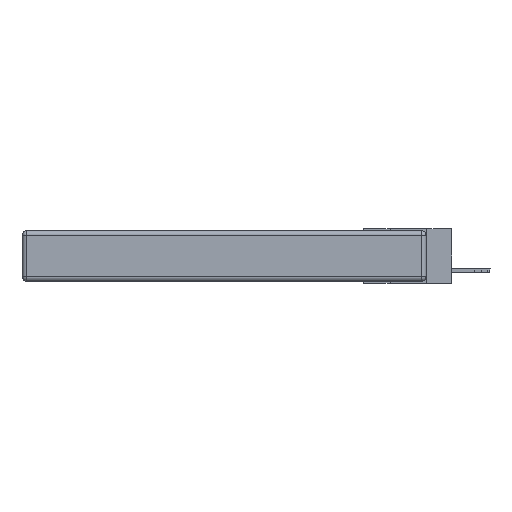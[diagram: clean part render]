
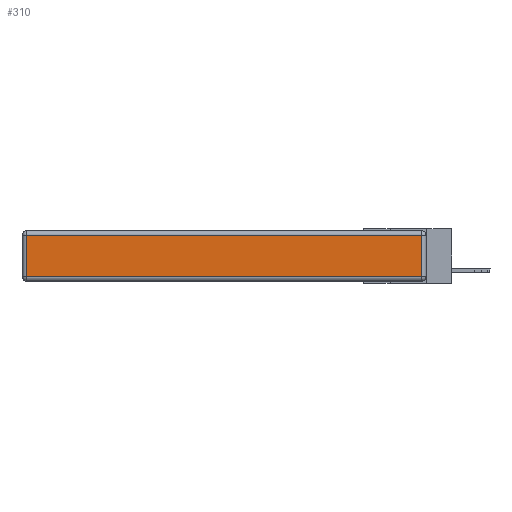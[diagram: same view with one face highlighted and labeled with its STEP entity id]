
A CAD part, left-side view. The second image highlights one B-rep face of the part: STEP entity #310.
In plain terms, the highlighted planar face has unit normal (-1, 0, 0).
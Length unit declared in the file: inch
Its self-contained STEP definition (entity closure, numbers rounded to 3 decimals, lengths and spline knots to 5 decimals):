
#116 = DIRECTION ( 'NONE',  ( 0., 1., 0. ) ) ;
#310 = ADVANCED_FACE ( 'NONE', ( #9126 ), #2979, .T. ) ;
#355 = DIRECTION ( 'NONE',  ( 0., 0., 1. ) ) ;
#733 = ORIENTED_EDGE ( 'NONE', *, *, #12509, .T. ) ;
#1388 = CARTESIAN_POINT ( 'NONE',  ( 0., 0.03, -0.03 ) ) ;
#1414 = ORIENTED_EDGE ( 'NONE', *, *, #11824, .T. ) ;
#1596 = VERTEX_POINT ( 'NONE', #8370 ) ;
#1909 = LINE ( 'NONE', #14400, #7045 ) ;
#2742 = CARTESIAN_POINT ( 'NONE',  ( 0., 0., -0.343 ) ) ;
#2979 = PLANE ( 'NONE',  #8669 ) ;
#3064 = EDGE_CURVE ( 'NONE', #5934, #12374, #6732, .T. ) ;
#3656 = CARTESIAN_POINT ( 'NONE',  ( 0., 2.72, -0.343 ) ) ;
#4066 = DIRECTION ( 'NONE',  ( -1., 0., 0. ) ) ;
#4663 = CARTESIAN_POINT ( 'NONE',  ( 0., 2.72, -0.03 ) ) ;
#4670 = ORIENTED_EDGE ( 'NONE', *, *, #5881, .T. ) ;
#5603 = LINE ( 'NONE', #5982, #16171 ) ;
#5881 = EDGE_CURVE ( 'NONE', #12374, #9298, #1909, .T. ) ;
#5934 = VERTEX_POINT ( 'NONE', #6815 ) ;
#5982 = CARTESIAN_POINT ( 'NONE',  ( 0., 0., -0.313 ) ) ;
#6732 = LINE ( 'NONE', #11136, #16640 ) ;
#6815 = CARTESIAN_POINT ( 'NONE',  ( 0., 0.03, -0.313 ) ) ;
#7045 = VECTOR ( 'NONE', #116, 39.37008 ) ;
#8370 = CARTESIAN_POINT ( 'NONE',  ( 0., 2.72, -0.313 ) ) ;
#8669 = AXIS2_PLACEMENT_3D ( 'NONE', #2742, #4066, #355 ) ;
#9126 = FACE_OUTER_BOUND ( 'NONE', #9827, .T. ) ;
#9298 = VERTEX_POINT ( 'NONE', #4663 ) ;
#9827 = EDGE_LOOP ( 'NONE', ( #1414, #11510, #4670, #733 ) ) ;
#9885 = VECTOR ( 'NONE', #15249, 39.37008 ) ;
#11136 = CARTESIAN_POINT ( 'NONE',  ( 0., 0.03, -0.343 ) ) ;
#11510 = ORIENTED_EDGE ( 'NONE', *, *, #3064, .T. ) ;
#11824 = EDGE_CURVE ( 'NONE', #1596, #5934, #5603, .T. ) ;
#12209 = DIRECTION ( 'NONE',  ( 0., 0., 1. ) ) ;
#12374 = VERTEX_POINT ( 'NONE', #1388 ) ;
#12509 = EDGE_CURVE ( 'NONE', #9298, #1596, #13704, .T. ) ;
#13158 = DIRECTION ( 'NONE',  ( 0., -1., 0. ) ) ;
#13704 = LINE ( 'NONE', #3656, #9885 ) ;
#14400 = CARTESIAN_POINT ( 'NONE',  ( 0., 2.75, -0.03 ) ) ;
#15249 = DIRECTION ( 'NONE',  ( 0., 0., -1. ) ) ;
#16171 = VECTOR ( 'NONE', #13158, 39.37008 ) ;
#16640 = VECTOR ( 'NONE', #12209, 39.37008 ) ;
